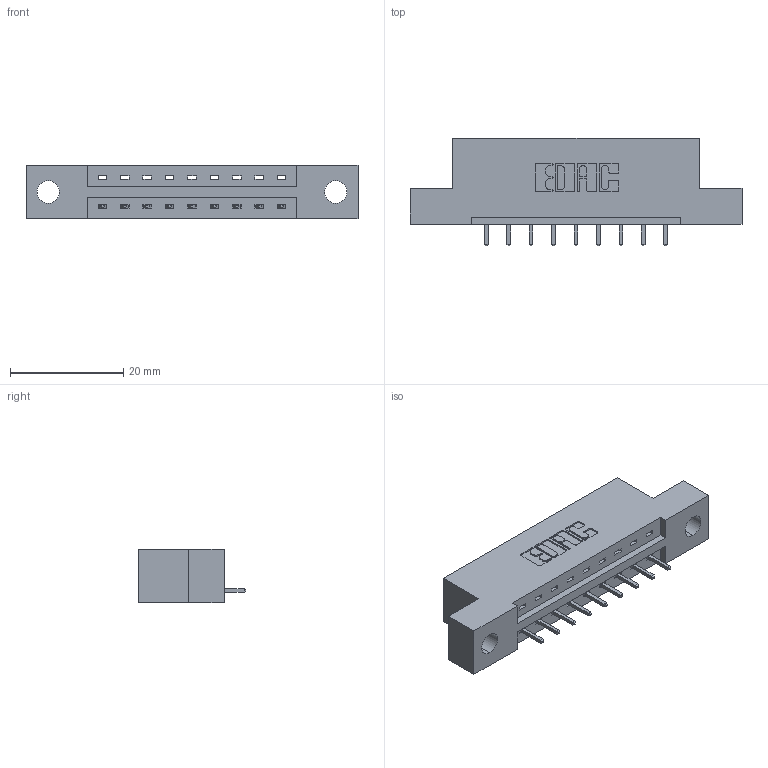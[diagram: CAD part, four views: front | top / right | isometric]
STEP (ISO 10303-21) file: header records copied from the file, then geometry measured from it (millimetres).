
FILE_DESCRIPTION (( 'STEP AP203' ), '1' );
FILE_NAME ('387-009-521-104.STEP', '2019-10-02T04:38:26', ( '' ), ( '' ), 'SwSTEP 2.0', 'SolidWorks 2016', '' );
FILE_SCHEMA (( 'CONFIG_CONTROL_DESIGN' ));
Length unit declared in the file: inch
Products named in the file (3): 387-009-521-104; 345-292-001_345-293-121; 337 Part_Flush Mounting Lugs - 0.156 Dia-TH
Assembly tree (10 placements, depth 2):
  387-009-521-104
    337 Part_Flush Mounting Lugs - 0.156 Dia-TH
    345-292-001_345-293-121  x9
Bounding box: 58.67 x 19.06 x 9.4 mm (x, y, z)
Volume: 5571.8 mm3; surface area: 5261.2 mm2
Topology: 10 solids, 10 shells, 672 faces, 2003 edges, 1322 vertices
Faces by surface type: plane 484, cylinder 188
Entity records: 10979 total; most frequent: CARTESIAN_POINT 1917, ORIENTED_EDGE 1862, DIRECTION 1681, EDGE_CURVE 931, LINE 803, VECTOR 803, VERTEX_POINT 618, AXIS2_PLACEMENT_3D 439
